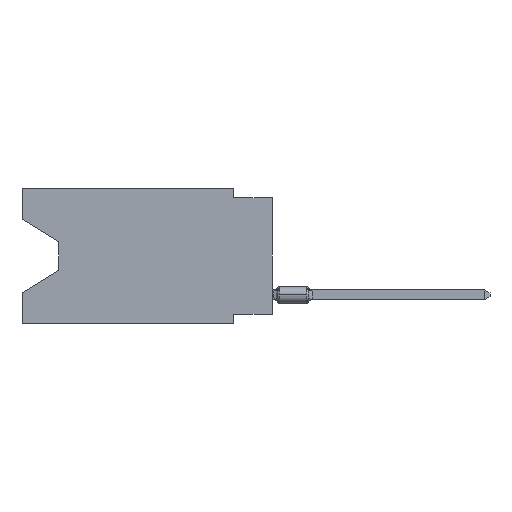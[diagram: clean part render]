
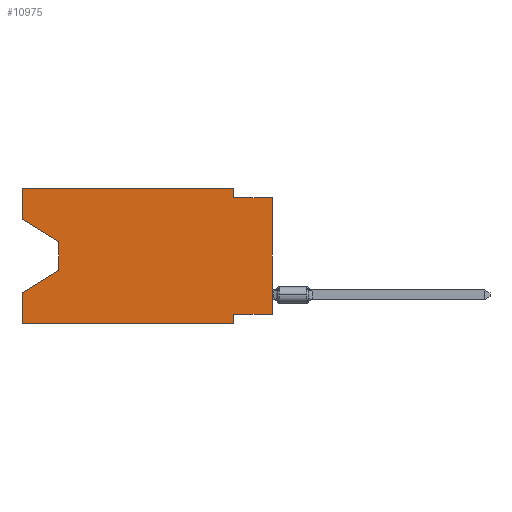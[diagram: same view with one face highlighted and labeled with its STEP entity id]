
A CAD part, left-side view. The second image highlights one B-rep face of the part: STEP entity #10975.
In plain terms, the highlighted planar face has unit normal (-1, 0, 0).
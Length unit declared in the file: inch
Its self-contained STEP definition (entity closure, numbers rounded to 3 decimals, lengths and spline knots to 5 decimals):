
#20 = ORIENTED_EDGE ( 'NONE', *, *, #5580, .F. ) ;
#99 = AXIS2_PLACEMENT_3D ( 'NONE', #15017, #8847, #18103 ) ;
#195 = VECTOR ( 'NONE', #14443, 39.37008 ) ;
#329 = DIRECTION ( 'NONE',  ( 0., 0., -1. ) ) ;
#691 = CARTESIAN_POINT ( 'NONE',  ( 0., 0.645, -0.08025 ) ) ;
#706 = EDGE_CURVE ( 'NONE', #17393, #16804, #14783, .T. ) ;
#914 = VECTOR ( 'NONE', #7214, 39.37008 ) ;
#934 = EDGE_LOOP ( 'NONE', ( #3239, #8054, #19426, #1328, #6267, #18263, #13657, #18837, #20, #11902, #8546, #9472 ) ) ;
#1158 = CARTESIAN_POINT ( 'NONE',  ( 0., 0., -0.325 ) ) ;
#1196 = DIRECTION ( 'NONE',  ( 0., -1., 0. ) ) ;
#1328 = ORIENTED_EDGE ( 'NONE', *, *, #18956, .F. ) ;
#1509 = DIRECTION ( 'NONE',  ( 0., 0., 1. ) ) ;
#1747 = CARTESIAN_POINT ( 'NONE',  ( 0., 0.55, -0.212 ) ) ;
#2419 = DIRECTION ( 'NONE',  ( 0., 0., 1. ) ) ;
#3223 = VECTOR ( 'NONE', #3654, 39.37008 ) ;
#3239 = ORIENTED_EDGE ( 'NONE', *, *, #15869, .T. ) ;
#3247 = EDGE_CURVE ( 'NONE', #12422, #15219, #16699, .T. ) ;
#3654 = DIRECTION ( 'NONE',  ( 0., 0., 1. ) ) ;
#4259 = DIRECTION ( 'NONE',  ( 0., 0., -1. ) ) ;
#4362 = PLANE ( 'NONE',  #99 ) ;
#4623 = CARTESIAN_POINT ( 'NONE',  ( 0., 0.55, -0.138 ) ) ;
#4657 = CARTESIAN_POINT ( 'NONE',  ( 0., 0.645, -0.35 ) ) ;
#5015 = CARTESIAN_POINT ( 'NONE',  ( 0., 0.1, -0.025 ) ) ;
#5174 = CARTESIAN_POINT ( 'NONE',  ( 0., 0.55, -0.212 ) ) ;
#5355 = LINE ( 'NONE', #11633, #3223 ) ;
#5374 = CARTESIAN_POINT ( 'NONE',  ( 0., 0.1, 0. ) ) ;
#5580 = EDGE_CURVE ( 'NONE', #9855, #17991, #15582, .T. ) ;
#5900 = CARTESIAN_POINT ( 'NONE',  ( 0., 0.645, 0. ) ) ;
#6093 = VECTOR ( 'NONE', #12469, 39.37008 ) ;
#6267 = ORIENTED_EDGE ( 'NONE', *, *, #3247, .T. ) ;
#7062 = VERTEX_POINT ( 'NONE', #5900 ) ;
#7214 = DIRECTION ( 'NONE',  ( 0., 1., 0. ) ) ;
#7349 = FACE_OUTER_BOUND ( 'NONE', #934, .T. ) ;
#7417 = LINE ( 'NONE', #1747, #17383 ) ;
#7478 = EDGE_CURVE ( 'NONE', #17393, #17991, #5355, .T. ) ;
#7620 = CARTESIAN_POINT ( 'NONE',  ( 0., 0., -0.025 ) ) ;
#7679 = LINE ( 'NONE', #15447, #6093 ) ;
#7693 = CARTESIAN_POINT ( 'NONE',  ( 0., 0., -0.325 ) ) ;
#7719 = EDGE_CURVE ( 'NONE', #10914, #7062, #14461, .T. ) ;
#7726 = VECTOR ( 'NONE', #1196, 39.37008 ) ;
#7965 = EDGE_CURVE ( 'NONE', #13791, #9855, #7679, .T. ) ;
#8054 = ORIENTED_EDGE ( 'NONE', *, *, #9744, .T. ) ;
#8536 = VECTOR ( 'NONE', #1509, 39.37008 ) ;
#8546 = ORIENTED_EDGE ( 'NONE', *, *, #11031, .F. ) ;
#8847 = DIRECTION ( 'NONE',  ( 1., 0., 0. ) ) ;
#8904 = VECTOR ( 'NONE', #10543, 39.37008 ) ;
#9472 = ORIENTED_EDGE ( 'NONE', *, *, #7719, .F. ) ;
#9615 = VECTOR ( 'NONE', #329, 39.37008 ) ;
#9669 = LINE ( 'NONE', #17326, #195 ) ;
#9744 = EDGE_CURVE ( 'NONE', #10720, #12493, #17898, .T. ) ;
#9855 = VERTEX_POINT ( 'NONE', #5015 ) ;
#10354 = EDGE_CURVE ( 'NONE', #16804, #15219, #15457, .T. ) ;
#10543 = DIRECTION ( 'NONE',  ( 0., -1., 0. ) ) ;
#10720 = VERTEX_POINT ( 'NONE', #11154 ) ;
#10910 = DIRECTION ( 'NONE',  ( 0., -1., 0. ) ) ;
#10914 = VERTEX_POINT ( 'NONE', #691 ) ;
#10975 = ADVANCED_FACE ( 'NONE', ( #7349 ), #4362, .F. ) ;
#11031 = EDGE_CURVE ( 'NONE', #7062, #13791, #13422, .T. ) ;
#11061 = VECTOR ( 'NONE', #10910, 39.37008 ) ;
#11154 = CARTESIAN_POINT ( 'NONE',  ( 0., 0.55, -0.138 ) ) ;
#11214 = CARTESIAN_POINT ( 'NONE',  ( 0., 0.645, -0.26975 ) ) ;
#11278 = CARTESIAN_POINT ( 'NONE',  ( 0., 0.645, 0. ) ) ;
#11633 = CARTESIAN_POINT ( 'NONE',  ( 0., 0., 0. ) ) ;
#11902 = ORIENTED_EDGE ( 'NONE', *, *, #7965, .F. ) ;
#12159 = VECTOR ( 'NONE', #4259, 39.37008 ) ;
#12422 = VERTEX_POINT ( 'NONE', #16929 ) ;
#12469 = DIRECTION ( 'NONE',  ( 0., 0., -1. ) ) ;
#12493 = VERTEX_POINT ( 'NONE', #5174 ) ;
#13422 = LINE ( 'NONE', #19690, #7726 ) ;
#13657 = ORIENTED_EDGE ( 'NONE', *, *, #706, .F. ) ;
#13791 = VERTEX_POINT ( 'NONE', #5374 ) ;
#13961 = CARTESIAN_POINT ( 'NONE',  ( 0., 0.1, -0.35 ) ) ;
#14443 = DIRECTION ( 'NONE',  ( 0., -0.855, -0.519 ) ) ;
#14461 = LINE ( 'NONE', #11278, #19455 ) ;
#14564 = VERTEX_POINT ( 'NONE', #11214 ) ;
#14783 = LINE ( 'NONE', #1158, #914 ) ;
#14889 = CARTESIAN_POINT ( 'NONE',  ( 0., 0.1, -0.325 ) ) ;
#15017 = CARTESIAN_POINT ( 'NONE',  ( 0., 0.645, 0. ) ) ;
#15219 = VERTEX_POINT ( 'NONE', #16687 ) ;
#15243 = CARTESIAN_POINT ( 'NONE',  ( 0., 0.645, 0. ) ) ;
#15447 = CARTESIAN_POINT ( 'NONE',  ( 0., 0.1, 0. ) ) ;
#15457 = LINE ( 'NONE', #13961, #9615 ) ;
#15582 = LINE ( 'NONE', #7620, #11061 ) ;
#15869 = EDGE_CURVE ( 'NONE', #10914, #10720, #9669, .T. ) ;
#15894 = CARTESIAN_POINT ( 'NONE',  ( 0., 0., -0.025 ) ) ;
#16687 = CARTESIAN_POINT ( 'NONE',  ( 0., 0.1, -0.35 ) ) ;
#16699 = LINE ( 'NONE', #4657, #8904 ) ;
#16804 = VERTEX_POINT ( 'NONE', #14889 ) ;
#16824 = LINE ( 'NONE', #15243, #8536 ) ;
#16869 = DIRECTION ( 'NONE',  ( 0., 0.855, -0.519 ) ) ;
#16929 = CARTESIAN_POINT ( 'NONE',  ( 0., 0.645, -0.35 ) ) ;
#16990 = EDGE_CURVE ( 'NONE', #12493, #14564, #7417, .T. ) ;
#17326 = CARTESIAN_POINT ( 'NONE',  ( 0., 0.645, -0.08025 ) ) ;
#17383 = VECTOR ( 'NONE', #16869, 39.37008 ) ;
#17393 = VERTEX_POINT ( 'NONE', #7693 ) ;
#17898 = LINE ( 'NONE', #4623, #12159 ) ;
#17991 = VERTEX_POINT ( 'NONE', #15894 ) ;
#18103 = DIRECTION ( 'NONE',  ( 0., 0., -1. ) ) ;
#18263 = ORIENTED_EDGE ( 'NONE', *, *, #10354, .F. ) ;
#18837 = ORIENTED_EDGE ( 'NONE', *, *, #7478, .T. ) ;
#18956 = EDGE_CURVE ( 'NONE', #12422, #14564, #16824, .T. ) ;
#19426 = ORIENTED_EDGE ( 'NONE', *, *, #16990, .T. ) ;
#19455 = VECTOR ( 'NONE', #2419, 39.37008 ) ;
#19690 = CARTESIAN_POINT ( 'NONE',  ( 0., 0.645, 0. ) ) ;
